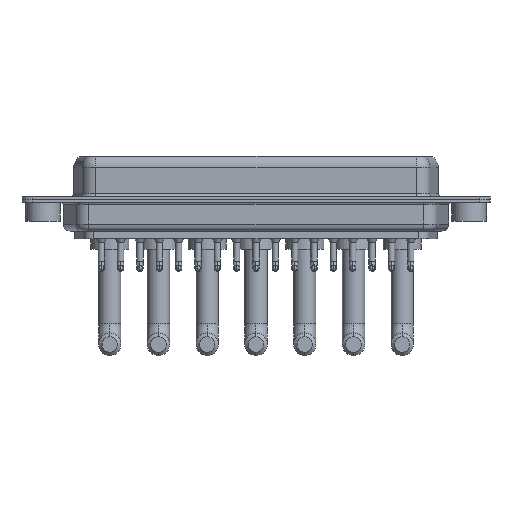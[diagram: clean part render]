
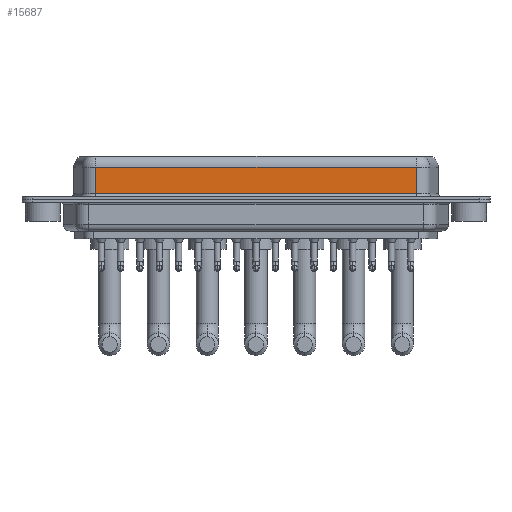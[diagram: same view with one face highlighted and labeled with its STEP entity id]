
A CAD part, front view. The second image highlights one B-rep face of the part: STEP entity #15687.
In plain terms, the highlighted planar face has unit normal (0, -1, 0).
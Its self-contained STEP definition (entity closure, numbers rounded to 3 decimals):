
#544 = ORIENTED_EDGE ( 'NONE', *, *, #7668, .F. ) ;
#742 = VERTEX_POINT ( 'NONE', #907 ) ;
#907 = CARTESIAN_POINT ( 'NONE',  ( 53.41, -5.375, 4.65 ) ) ;
#946 = DIRECTION ( 'NONE',  ( 0., 1., 0. ) ) ;
#1024 = EDGE_CURVE ( 'NONE', #742, #10600, #10157, .T. ) ;
#2088 = VECTOR ( 'NONE', #16710, 1000. ) ;
#2682 = EDGE_LOOP ( 'NONE', ( #544, #17104, #5659, #6576 ) ) ;
#3634 = VERTEX_POINT ( 'NONE', #13803 ) ;
#5659 = ORIENTED_EDGE ( 'NONE', *, *, #11345, .T. ) ;
#6307 = DIRECTION ( 'NONE',  ( 0., 0., 1. ) ) ;
#6576 = ORIENTED_EDGE ( 'NONE', *, *, #13603, .T. ) ;
#7668 = EDGE_CURVE ( 'NONE', #742, #9811, #20865, .T. ) ;
#8700 = CARTESIAN_POINT ( 'NONE',  ( 53.41, -5.375, 0.9 ) ) ;
#9173 = LINE ( 'NONE', #16948, #12951 ) ;
#9811 = VERTEX_POINT ( 'NONE', #16641 ) ;
#10157 = LINE ( 'NONE', #16605, #2088 ) ;
#10430 = LINE ( 'NONE', #8700, #15058 ) ;
#10600 = VERTEX_POINT ( 'NONE', #14638 ) ;
#11345 = EDGE_CURVE ( 'NONE', #10600, #3634, #9173, .T. ) ;
#12698 = CARTESIAN_POINT ( 'NONE',  ( 53.41, -5.375, 6.4 ) ) ;
#12776 = FACE_OUTER_BOUND ( 'NONE', #2682, .T. ) ;
#12951 = VECTOR ( 'NONE', #17339, 1000. ) ;
#13149 = VECTOR ( 'NONE', #13886, 1000. ) ;
#13437 = DIRECTION ( 'NONE',  ( 1., 0., 0. ) ) ;
#13603 = EDGE_CURVE ( 'NONE', #3634, #9811, #10430, .T. ) ;
#13803 = CARTESIAN_POINT ( 'NONE',  ( 7.59, -5.375, 0.9 ) ) ;
#13886 = DIRECTION ( 'NONE',  ( 0., 0., -1. ) ) ;
#14638 = CARTESIAN_POINT ( 'NONE',  ( 7.59, -5.375, 4.65 ) ) ;
#15058 = VECTOR ( 'NONE', #13437, 1000. ) ;
#15687 = ADVANCED_FACE ( 'NONE', ( #12776 ), #15909, .F. ) ;
#15909 = PLANE ( 'NONE',  #18919 ) ;
#16605 = CARTESIAN_POINT ( 'NONE',  ( 53.41, -5.375, 4.65 ) ) ;
#16641 = CARTESIAN_POINT ( 'NONE',  ( 53.41, -5.375, 0.9 ) ) ;
#16710 = DIRECTION ( 'NONE',  ( -1., 0., 0. ) ) ;
#16948 = CARTESIAN_POINT ( 'NONE',  ( 7.59, -5.375, 6.4 ) ) ;
#17104 = ORIENTED_EDGE ( 'NONE', *, *, #1024, .T. ) ;
#17339 = DIRECTION ( 'NONE',  ( 0., 0., -1. ) ) ;
#17616 = CARTESIAN_POINT ( 'NONE',  ( 53.41, -5.375, 6.4 ) ) ;
#18919 = AXIS2_PLACEMENT_3D ( 'NONE', #17616, #946, #6307 ) ;
#20865 = LINE ( 'NONE', #12698, #13149 ) ;
